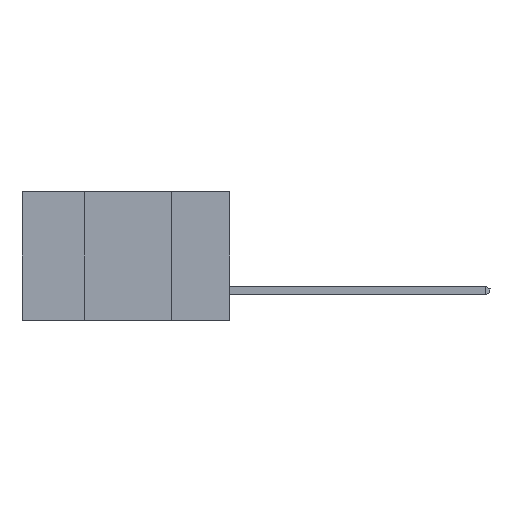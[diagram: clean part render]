
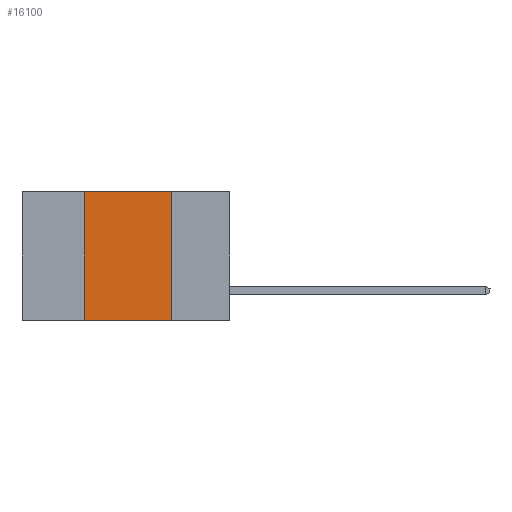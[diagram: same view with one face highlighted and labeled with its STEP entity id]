
A CAD part, left-side view. The second image highlights one B-rep face of the part: STEP entity #16100.
In plain terms, the highlighted planar face has unit normal (-1, 0, 0).
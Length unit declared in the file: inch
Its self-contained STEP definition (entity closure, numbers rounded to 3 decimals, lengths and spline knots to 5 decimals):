
#289 = LINE ( 'NONE', #9952, #6695 ) ;
#837 = ORIENTED_EDGE ( 'NONE', *, *, #10653, .F. ) ;
#1057 = DIRECTION ( 'NONE',  ( 0., 0., -1. ) ) ;
#2100 = ORIENTED_EDGE ( 'NONE', *, *, #8664, .F. ) ;
#2138 = PLANE ( 'NONE',  #16470 ) ;
#2297 = ORIENTED_EDGE ( 'NONE', *, *, #12327, .F. ) ;
#4467 = ORIENTED_EDGE ( 'NONE', *, *, #9240, .T. ) ;
#4536 = VECTOR ( 'NONE', #14176, 39.37008 ) ;
#5880 = CARTESIAN_POINT ( 'NONE',  ( 0., 0.17, 0. ) ) ;
#6106 = VERTEX_POINT ( 'NONE', #15760 ) ;
#6213 = CARTESIAN_POINT ( 'NONE',  ( 0., 0.42, 0. ) ) ;
#6486 = VERTEX_POINT ( 'NONE', #5880 ) ;
#6695 = VECTOR ( 'NONE', #15487, 39.37008 ) ;
#7551 = DIRECTION ( 'NONE',  ( 1., 0., 0. ) ) ;
#7813 = FACE_OUTER_BOUND ( 'NONE', #10436, .T. ) ;
#8181 = LINE ( 'NONE', #9350, #15249 ) ;
#8664 = EDGE_CURVE ( 'NONE', #16143, #6486, #289, .T. ) ;
#9166 = DIRECTION ( 'NONE',  ( 0., 0., -1. ) ) ;
#9240 = EDGE_CURVE ( 'NONE', #6106, #9447, #10550, .T. ) ;
#9350 = CARTESIAN_POINT ( 'NONE',  ( 0., 0.17, -0.37 ) ) ;
#9447 = VERTEX_POINT ( 'NONE', #15248 ) ;
#9628 = LINE ( 'NONE', #15344, #4536 ) ;
#9952 = CARTESIAN_POINT ( 'NONE',  ( 0., 0.6, 0. ) ) ;
#10436 = EDGE_LOOP ( 'NONE', ( #2297, #2100, #837, #4467 ) ) ;
#10464 = VECTOR ( 'NONE', #10726, 39.37008 ) ;
#10550 = LINE ( 'NONE', #16088, #10464 ) ;
#10653 = EDGE_CURVE ( 'NONE', #6106, #16143, #9628, .T. ) ;
#10726 = DIRECTION ( 'NONE',  ( 0., -1., 0. ) ) ;
#12327 = EDGE_CURVE ( 'NONE', #6486, #9447, #8181, .T. ) ;
#13265 = CARTESIAN_POINT ( 'NONE',  ( 0., 0.6, 0. ) ) ;
#14176 = DIRECTION ( 'NONE',  ( 0., 0., 1. ) ) ;
#15248 = CARTESIAN_POINT ( 'NONE',  ( 0., 0.17, -0.37 ) ) ;
#15249 = VECTOR ( 'NONE', #1057, 39.37008 ) ;
#15344 = CARTESIAN_POINT ( 'NONE',  ( 0., 0.42, -0.37 ) ) ;
#15487 = DIRECTION ( 'NONE',  ( 0., -1., 0. ) ) ;
#15760 = CARTESIAN_POINT ( 'NONE',  ( 0., 0.42, -0.37 ) ) ;
#16088 = CARTESIAN_POINT ( 'NONE',  ( 0., 0.6, -0.37 ) ) ;
#16100 = ADVANCED_FACE ( 'NONE', ( #7813 ), #2138, .F. ) ;
#16143 = VERTEX_POINT ( 'NONE', #6213 ) ;
#16470 = AXIS2_PLACEMENT_3D ( 'NONE', #13265, #7551, #9166 ) ;
